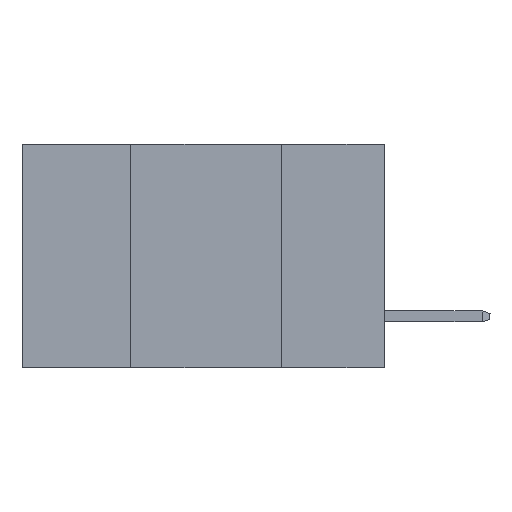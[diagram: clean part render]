
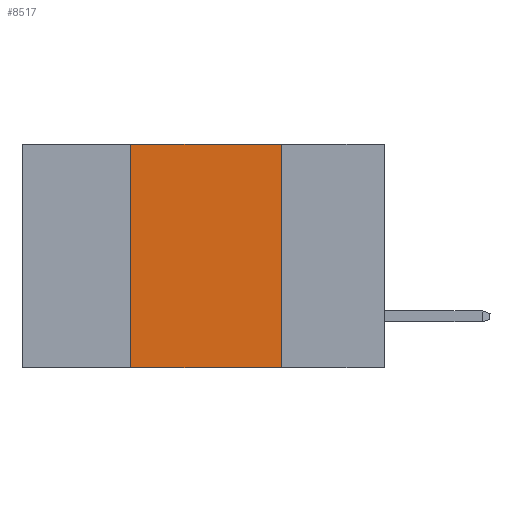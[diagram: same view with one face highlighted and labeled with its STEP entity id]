
A CAD part, left-side view. The second image highlights one B-rep face of the part: STEP entity #8517.
In plain terms, the highlighted planar face has unit normal (-1, 0, 0).
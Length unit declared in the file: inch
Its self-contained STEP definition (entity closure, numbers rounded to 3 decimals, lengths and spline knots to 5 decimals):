
#317 = VERTEX_POINT ( 'NONE', #1810 ) ;
#1136 = DIRECTION ( 'NONE',  ( 0., 0., -1. ) ) ;
#1250 = LINE ( 'NONE', #10686, #5230 ) ;
#1336 = VECTOR ( 'NONE', #13889, 39.37008 ) ;
#1587 = DIRECTION ( 'NONE',  ( 0., -1., 0. ) ) ;
#1810 = CARTESIAN_POINT ( 'NONE',  ( 0., 0.17, -0.37 ) ) ;
#2331 = PLANE ( 'NONE',  #5312 ) ;
#2486 = DIRECTION ( 'NONE',  ( 0., 0., 1. ) ) ;
#3120 = LINE ( 'NONE', #9904, #1336 ) ;
#3970 = EDGE_CURVE ( 'NONE', #5910, #16074, #1250, .T. ) ;
#4061 = EDGE_CURVE ( 'NONE', #5910, #317, #13600, .T. ) ;
#4901 = EDGE_CURVE ( 'NONE', #16074, #14212, #3120, .T. ) ;
#4963 = CARTESIAN_POINT ( 'NONE',  ( 0., 0.17, 0. ) ) ;
#5230 = VECTOR ( 'NONE', #2486, 39.37008 ) ;
#5312 = AXIS2_PLACEMENT_3D ( 'NONE', #14609, #16117, #13462 ) ;
#5910 = VERTEX_POINT ( 'NONE', #7650 ) ;
#7137 = ORIENTED_EDGE ( 'NONE', *, *, #4901, .F. ) ;
#7650 = CARTESIAN_POINT ( 'NONE',  ( 0., 0.42, -0.37 ) ) ;
#8087 = CARTESIAN_POINT ( 'NONE',  ( 0., 0.17, -0.37 ) ) ;
#8517 = ADVANCED_FACE ( 'NONE', ( #9476 ), #2331, .F. ) ;
#9180 = VECTOR ( 'NONE', #1587, 39.37008 ) ;
#9476 = FACE_OUTER_BOUND ( 'NONE', #11326, .T. ) ;
#9501 = EDGE_CURVE ( 'NONE', #14212, #317, #13570, .T. ) ;
#9572 = VECTOR ( 'NONE', #1136, 39.37008 ) ;
#9882 = CARTESIAN_POINT ( 'NONE',  ( 0., 0.6, -0.37 ) ) ;
#9904 = CARTESIAN_POINT ( 'NONE',  ( 0., 0.6, 0. ) ) ;
#10371 = ORIENTED_EDGE ( 'NONE', *, *, #3970, .F. ) ;
#10686 = CARTESIAN_POINT ( 'NONE',  ( 0., 0.42, -0.37 ) ) ;
#11326 = EDGE_LOOP ( 'NONE', ( #14158, #7137, #10371, #13083 ) ) ;
#12264 = CARTESIAN_POINT ( 'NONE',  ( 0., 0.42, 0. ) ) ;
#13083 = ORIENTED_EDGE ( 'NONE', *, *, #4061, .T. ) ;
#13462 = DIRECTION ( 'NONE',  ( 0., 0., -1. ) ) ;
#13570 = LINE ( 'NONE', #8087, #9572 ) ;
#13600 = LINE ( 'NONE', #9882, #9180 ) ;
#13889 = DIRECTION ( 'NONE',  ( 0., -1., 0. ) ) ;
#14158 = ORIENTED_EDGE ( 'NONE', *, *, #9501, .F. ) ;
#14212 = VERTEX_POINT ( 'NONE', #4963 ) ;
#14609 = CARTESIAN_POINT ( 'NONE',  ( 0., 0.6, 0. ) ) ;
#16074 = VERTEX_POINT ( 'NONE', #12264 ) ;
#16117 = DIRECTION ( 'NONE',  ( 1., 0., 0. ) ) ;
